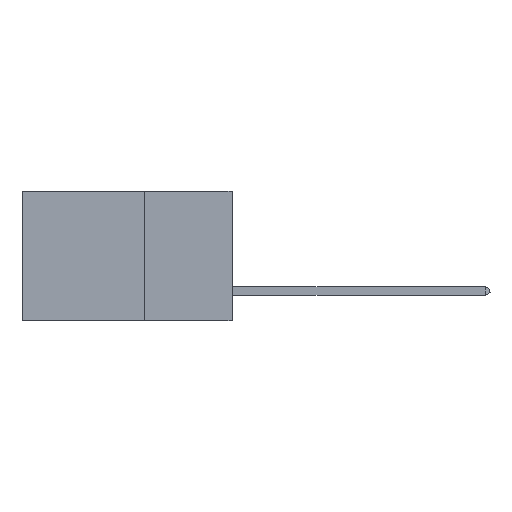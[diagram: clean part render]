
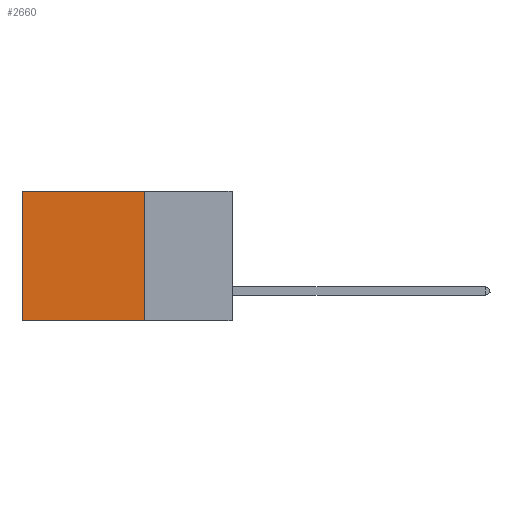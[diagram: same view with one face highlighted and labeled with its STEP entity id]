
A CAD part, left-side view. The second image highlights one B-rep face of the part: STEP entity #2660.
In plain terms, the highlighted planar face has unit normal (-1, 0, 0).
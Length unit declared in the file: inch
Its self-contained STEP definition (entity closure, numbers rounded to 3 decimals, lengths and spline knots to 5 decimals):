
#648 = ORIENTED_EDGE ( 'NONE', *, *, #11543, .F. ) ;
#653 = VECTOR ( 'NONE', #5991, 39.37008 ) ;
#685 = CARTESIAN_POINT ( 'NONE',  ( 0.2875, 0.25, -0.37 ) ) ;
#2054 = CARTESIAN_POINT ( 'NONE',  ( 0.2875, 0.6, 0. ) ) ;
#2660 = ADVANCED_FACE ( 'NONE', ( #3359 ), #20682, .F. ) ;
#3359 = FACE_OUTER_BOUND ( 'NONE', #17815, .T. ) ;
#3817 = EDGE_CURVE ( 'NONE', #8819, #9584, #3893, .T. ) ;
#3823 = VERTEX_POINT ( 'NONE', #7959 ) ;
#3893 = LINE ( 'NONE', #5820, #18039 ) ;
#4220 = ORIENTED_EDGE ( 'NONE', *, *, #3817, .F. ) ;
#4958 = DIRECTION ( 'NONE',  ( 1., 0., 0. ) ) ;
#5584 = DIRECTION ( 'NONE',  ( 0., 0., -1. ) ) ;
#5820 = CARTESIAN_POINT ( 'NONE',  ( 0.2875, 0.25, 0. ) ) ;
#5991 = DIRECTION ( 'NONE',  ( 0., 1., 0. ) ) ;
#6141 = DIRECTION ( 'NONE',  ( 0., 1., 0. ) ) ;
#7959 = CARTESIAN_POINT ( 'NONE',  ( 0.2875, 0.6, 0. ) ) ;
#8125 = DIRECTION ( 'NONE',  ( 0., 0., -1. ) ) ;
#8819 = VERTEX_POINT ( 'NONE', #11589 ) ;
#8892 = CARTESIAN_POINT ( 'NONE',  ( 0.2875, 0.25, 0. ) ) ;
#9584 = VERTEX_POINT ( 'NONE', #685 ) ;
#9599 = VECTOR ( 'NONE', #6141, 39.37008 ) ;
#10225 = ORIENTED_EDGE ( 'NONE', *, *, #22117, .T. ) ;
#11543 = EDGE_CURVE ( 'NONE', #9584, #25126, #21192, .T. ) ;
#11589 = CARTESIAN_POINT ( 'NONE',  ( 0.2875, 0.25, 0. ) ) ;
#11760 = CARTESIAN_POINT ( 'NONE',  ( 0.2875, 0.6, -0.37 ) ) ;
#16331 = VECTOR ( 'NONE', #5584, 39.37008 ) ;
#17058 = ORIENTED_EDGE ( 'NONE', *, *, #19846, .T. ) ;
#17760 = AXIS2_PLACEMENT_3D ( 'NONE', #8892, #4958, #18814 ) ;
#17815 = EDGE_LOOP ( 'NONE', ( #10225, #648, #4220, #17058 ) ) ;
#18039 = VECTOR ( 'NONE', #8125, 39.37008 ) ;
#18187 = CARTESIAN_POINT ( 'NONE',  ( 0.2875, 0.25, 0. ) ) ;
#18517 = LINE ( 'NONE', #2054, #16331 ) ;
#18814 = DIRECTION ( 'NONE',  ( 0., 0., -1. ) ) ;
#18920 = LINE ( 'NONE', #18187, #9599 ) ;
#19768 = CARTESIAN_POINT ( 'NONE',  ( 0.2875, 0.25, -0.37 ) ) ;
#19846 = EDGE_CURVE ( 'NONE', #8819, #3823, #18920, .T. ) ;
#20682 = PLANE ( 'NONE',  #17760 ) ;
#21192 = LINE ( 'NONE', #19768, #653 ) ;
#22117 = EDGE_CURVE ( 'NONE', #3823, #25126, #18517, .T. ) ;
#25126 = VERTEX_POINT ( 'NONE', #11760 ) ;
